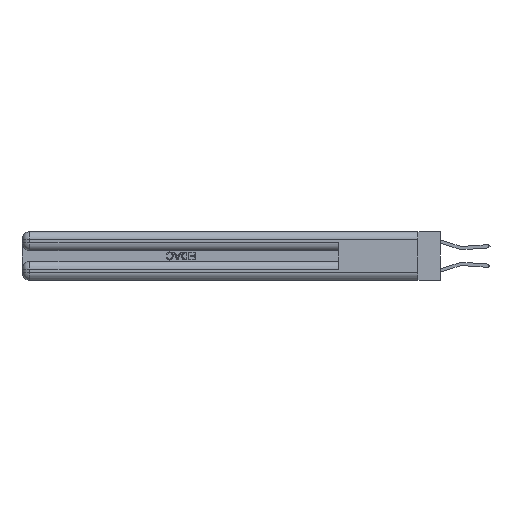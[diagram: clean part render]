
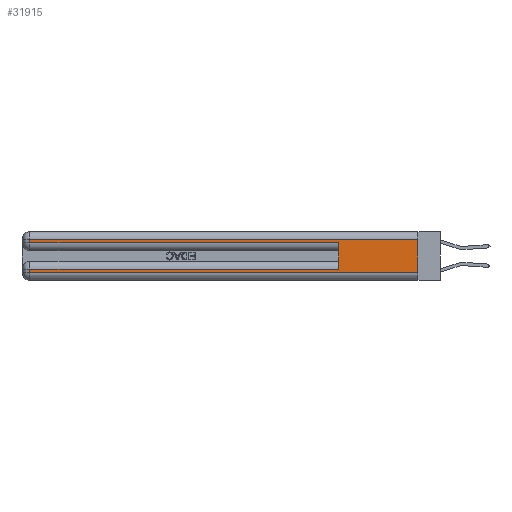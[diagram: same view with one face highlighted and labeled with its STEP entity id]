
A CAD part, left-side view. The second image highlights one B-rep face of the part: STEP entity #31915.
In plain terms, the highlighted planar face has unit normal (-1, 0, 0).
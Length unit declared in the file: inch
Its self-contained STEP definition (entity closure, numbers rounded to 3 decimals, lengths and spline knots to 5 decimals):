
#353 = CARTESIAN_POINT ( 'NONE',  ( 0., 0.6, 0.145 ) ) ;
#389 = LINE ( 'NONE', #27180, #7153 ) ;
#527 = CARTESIAN_POINT ( 'NONE',  ( 0., 2.94, 0.37 ) ) ;
#2065 = VERTEX_POINT ( 'NONE', #18616 ) ;
#2540 = CARTESIAN_POINT ( 'NONE',  ( 0., 2.94, 0.37 ) ) ;
#2994 = EDGE_CURVE ( 'NONE', #2065, #25833, #389, .T. ) ;
#3266 = EDGE_CURVE ( 'NONE', #6107, #25833, #28187, .T. ) ;
#3268 = CARTESIAN_POINT ( 'NONE',  ( 0., 2.94, 0.06 ) ) ;
#3455 = DIRECTION ( 'NONE',  ( 0., 0., -1. ) ) ;
#3711 = ORIENTED_EDGE ( 'NONE', *, *, #19439, .T. ) ;
#4696 = VECTOR ( 'NONE', #11104, 39.37008 ) ;
#4818 = DIRECTION ( 'NONE',  ( 0., -1., 0. ) ) ;
#5572 = LINE ( 'NONE', #13822, #4696 ) ;
#6043 = ORIENTED_EDGE ( 'NONE', *, *, #6576, .T. ) ;
#6107 = VERTEX_POINT ( 'NONE', #28684 ) ;
#6576 = EDGE_CURVE ( 'NONE', #28712, #2065, #16167, .T. ) ;
#6991 = CARTESIAN_POINT ( 'NONE',  ( 0., 2.94, 0.31 ) ) ;
#7153 = VECTOR ( 'NONE', #4818, 39.37008 ) ;
#7544 = LINE ( 'NONE', #31100, #36448 ) ;
#7686 = DIRECTION ( 'NONE',  ( 0., 1., 0. ) ) ;
#8157 = CARTESIAN_POINT ( 'NONE',  ( 0., 0., 0.06 ) ) ;
#8606 = VECTOR ( 'NONE', #30591, 39.37008 ) ;
#8685 = VECTOR ( 'NONE', #3455, 39.37008 ) ;
#9466 = DIRECTION ( 'NONE',  ( 0., 0., -1. ) ) ;
#9664 = EDGE_CURVE ( 'NONE', #29462, #30750, #16113, .T. ) ;
#10131 = ORIENTED_EDGE ( 'NONE', *, *, #3266, .F. ) ;
#11104 = DIRECTION ( 'NONE',  ( 0., 1., 0. ) ) ;
#12207 = PLANE ( 'NONE',  #26440 ) ;
#12686 = FACE_OUTER_BOUND ( 'NONE', #30949, .T. ) ;
#13822 = CARTESIAN_POINT ( 'NONE',  ( 0., 0., 0.31 ) ) ;
#14353 = DIRECTION ( 'NONE',  ( 0., 0., -1. ) ) ;
#15113 = CARTESIAN_POINT ( 'NONE',  ( 0., 0.6, 0.285 ) ) ;
#15288 = VECTOR ( 'NONE', #16693, 39.37008 ) ;
#15489 = LINE ( 'NONE', #24504, #31228 ) ;
#16113 = LINE ( 'NONE', #8157, #8606 ) ;
#16167 = LINE ( 'NONE', #2540, #15288 ) ;
#16200 = LINE ( 'NONE', #527, #8685 ) ;
#16312 = ORIENTED_EDGE ( 'NONE', *, *, #25760, .T. ) ;
#16693 = DIRECTION ( 'NONE',  ( 0., 0., -1. ) ) ;
#18616 = CARTESIAN_POINT ( 'NONE',  ( 0., 2.94, 0.285 ) ) ;
#19439 = EDGE_CURVE ( 'NONE', #6107, #25068, #15489, .T. ) ;
#20207 = DIRECTION ( 'NONE',  ( 0., 0., 1. ) ) ;
#20920 = ORIENTED_EDGE ( 'NONE', *, *, #2994, .T. ) ;
#22491 = EDGE_CURVE ( 'NONE', #30254, #30750, #7544, .T. ) ;
#23474 = CARTESIAN_POINT ( 'NONE',  ( 0., 0., 0.37 ) ) ;
#24504 = CARTESIAN_POINT ( 'NONE',  ( 0., 0., 0.085 ) ) ;
#25068 = VERTEX_POINT ( 'NONE', #35554 ) ;
#25760 = EDGE_CURVE ( 'NONE', #25068, #29462, #16200, .T. ) ;
#25833 = VERTEX_POINT ( 'NONE', #15113 ) ;
#26270 = DIRECTION ( 'NONE',  ( 1., 0., 0. ) ) ;
#26440 = AXIS2_PLACEMENT_3D ( 'NONE', #23474, #26270, #9466 ) ;
#26561 = VECTOR ( 'NONE', #20207, 39.37008 ) ;
#27180 = CARTESIAN_POINT ( 'NONE',  ( 0., 0., 0.285 ) ) ;
#28187 = LINE ( 'NONE', #353, #26561 ) ;
#28662 = CARTESIAN_POINT ( 'NONE',  ( 0., 0., 0.06 ) ) ;
#28684 = CARTESIAN_POINT ( 'NONE',  ( 0., 0.6, 0.085 ) ) ;
#28712 = VERTEX_POINT ( 'NONE', #6991 ) ;
#29083 = CARTESIAN_POINT ( 'NONE',  ( 0., 0., 0.31 ) ) ;
#29462 = VERTEX_POINT ( 'NONE', #3268 ) ;
#29640 = ORIENTED_EDGE ( 'NONE', *, *, #31669, .T. ) ;
#29671 = ORIENTED_EDGE ( 'NONE', *, *, #9664, .T. ) ;
#30254 = VERTEX_POINT ( 'NONE', #29083 ) ;
#30591 = DIRECTION ( 'NONE',  ( 0., -1., 0. ) ) ;
#30750 = VERTEX_POINT ( 'NONE', #28662 ) ;
#30949 = EDGE_LOOP ( 'NONE', ( #31306, #29640, #6043, #20920, #10131, #3711, #16312, #29671 ) ) ;
#31100 = CARTESIAN_POINT ( 'NONE',  ( 0., 0., 0.37 ) ) ;
#31228 = VECTOR ( 'NONE', #7686, 39.37008 ) ;
#31306 = ORIENTED_EDGE ( 'NONE', *, *, #22491, .F. ) ;
#31669 = EDGE_CURVE ( 'NONE', #30254, #28712, #5572, .T. ) ;
#31915 = ADVANCED_FACE ( 'NONE', ( #12686 ), #12207, .F. ) ;
#35554 = CARTESIAN_POINT ( 'NONE',  ( 0., 2.94, 0.085 ) ) ;
#36448 = VECTOR ( 'NONE', #14353, 39.37008 ) ;
